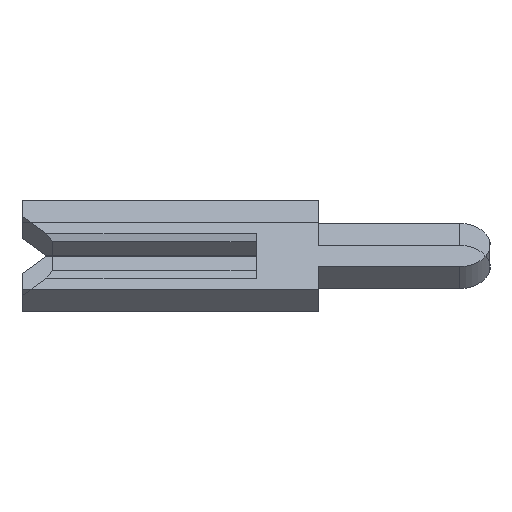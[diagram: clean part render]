
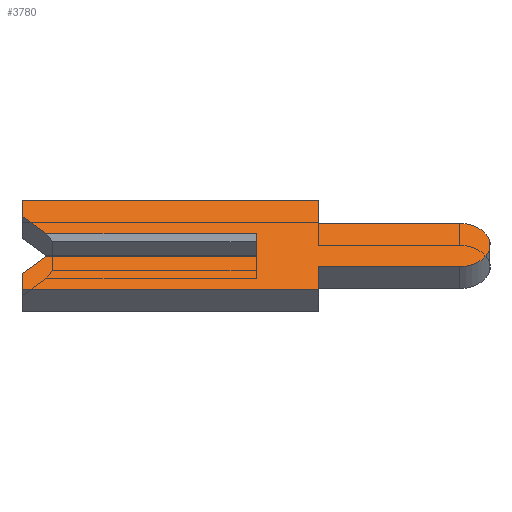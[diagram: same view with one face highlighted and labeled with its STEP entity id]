
A CAD part, left-side view. The second image highlights one B-rep face of the part: STEP entity #3780.
In plain terms, the highlighted face is planar.
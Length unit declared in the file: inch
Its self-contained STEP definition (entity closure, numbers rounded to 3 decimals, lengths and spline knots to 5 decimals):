
#26 = ORIENTED_EDGE ( 'NONE', *, *, #160, .F. ) ;
#28 = VECTOR ( 'NONE', #3910, 39.37008 ) ;
#71 = ORIENTED_EDGE ( 'NONE', *, *, #3265, .F. ) ;
#127 = ORIENTED_EDGE ( 'NONE', *, *, #2620, .F. ) ;
#139 = LINE ( 'NONE', #2826, #3987 ) ;
#149 = LINE ( 'NONE', #206, #2885 ) ;
#160 = EDGE_CURVE ( 'NONE', #2735, #2864, #1687, .T. ) ;
#175 = VECTOR ( 'NONE', #2562, 39.37008 ) ;
#206 = CARTESIAN_POINT ( 'NONE',  ( -0.01, -0.04, -0.0195 ) ) ;
#281 = CARTESIAN_POINT ( 'NONE',  ( -0.01, 0.1305, -0.0065 ) ) ;
#293 = DIRECTION ( 'NONE',  ( 0., -0.707, 0.707 ) ) ;
#316 = VERTEX_POINT ( 'NONE', #4026 ) ;
#367 = DIRECTION ( 'NONE',  ( 0., 0., -1. ) ) ;
#387 = LINE ( 'NONE', #1609, #175 ) ;
#411 = ORIENTED_EDGE ( 'NONE', *, *, #1567, .F. ) ;
#456 = VECTOR ( 'NONE', #2513, 39.37008 ) ;
#496 = VERTEX_POINT ( 'NONE', #1480 ) ;
#559 = DIRECTION ( 'NONE',  ( 0., 1., 0. ) ) ;
#669 = EDGE_CURVE ( 'NONE', #1331, #1097, #149, .T. ) ;
#706 = LINE ( 'NONE', #1332, #2945 ) ;
#759 = DIRECTION ( 'NONE',  ( 0., -1., 0. ) ) ;
#764 = EDGE_CURVE ( 'NONE', #1489, #2735, #1234, .T. ) ;
#836 = CARTESIAN_POINT ( 'NONE',  ( -0.01, -0.04, -0.04 ) ) ;
#882 = AXIS2_PLACEMENT_3D ( 'NONE', #1657, #1964, #367 ) ;
#922 = ORIENTED_EDGE ( 'NONE', *, *, #669, .F. ) ;
#923 = CARTESIAN_POINT ( 'NONE',  ( -0.01, 0.134, 0.01 ) ) ;
#948 = CARTESIAN_POINT ( 'NONE',  ( -0.01, 0., -0.01 ) ) ;
#951 = LINE ( 'NONE', #3582, #28 ) ;
#1019 = VERTEX_POINT ( 'NONE', #1838 ) ;
#1097 = VERTEX_POINT ( 'NONE', #1804 ) ;
#1100 = CARTESIAN_POINT ( 'NONE',  ( -0.01, 0.15, -0.026 ) ) ;
#1108 = LINE ( 'NONE', #1255, #3890 ) ;
#1149 = EDGE_CURVE ( 'NONE', #1521, #1019, #139, .T. ) ;
#1155 = ORIENTED_EDGE ( 'NONE', *, *, #1149, .T. ) ;
#1197 = DIRECTION ( 'NONE',  ( 0., -1., 0. ) ) ;
#1234 = LINE ( 'NONE', #3131, #1775 ) ;
#1255 = CARTESIAN_POINT ( 'NONE',  ( -0.01, 0.15, 0.04 ) ) ;
#1283 = ORIENTED_EDGE ( 'NONE', *, *, #2763, .F. ) ;
#1304 = LINE ( 'NONE', #1936, #3300 ) ;
#1317 = CARTESIAN_POINT ( 'NONE',  ( -0.01, 0.15, -0.04 ) ) ;
#1320 = VECTOR ( 'NONE', #293, 39.37008 ) ;
#1331 = VERTEX_POINT ( 'NONE', #2254 ) ;
#1332 = CARTESIAN_POINT ( 'NONE',  ( -0.01, -0.04, 0.04 ) ) ;
#1369 = DIRECTION ( 'NONE',  ( 0., 0., -1. ) ) ;
#1376 = DIRECTION ( 'NONE',  ( 0., 0., 1. ) ) ;
#1392 = EDGE_CURVE ( 'NONE', #496, #2068, #2881, .T. ) ;
#1480 = CARTESIAN_POINT ( 'NONE',  ( -0.01, 0.15, 0.026 ) ) ;
#1489 = VERTEX_POINT ( 'NONE', #836 ) ;
#1506 = EDGE_CURVE ( 'NONE', #2864, #2099, #3027, .T. ) ;
#1521 = VERTEX_POINT ( 'NONE', #923 ) ;
#1526 = CARTESIAN_POINT ( 'NONE',  ( -0.01, 0.15, 0.026 ) ) ;
#1539 = VERTEX_POINT ( 'NONE', #948 ) ;
#1567 = EDGE_CURVE ( 'NONE', #2068, #2023, #1108, .T. ) ;
#1589 = EDGE_CURVE ( 'NONE', #1097, #1489, #3474, .T. ) ;
#1609 = CARTESIAN_POINT ( 'NONE',  ( -0.01, 0.1305, 0.0065 ) ) ;
#1657 = CARTESIAN_POINT ( 'NONE',  ( -0.01, -0.1305, 0. ) ) ;
#1679 = VECTOR ( 'NONE', #2527, 39.37008 ) ;
#1687 = LINE ( 'NONE', #1100, #2042 ) ;
#1775 = VECTOR ( 'NONE', #2791, 39.37008 ) ;
#1804 = CARTESIAN_POINT ( 'NONE',  ( -0.01, -0.04, -0.0195 ) ) ;
#1817 = ORIENTED_EDGE ( 'NONE', *, *, #1506, .F. ) ;
#1837 = EDGE_CURVE ( 'NONE', #1539, #1019, #1304, .T. ) ;
#1838 = CARTESIAN_POINT ( 'NONE',  ( -0.01, 0., 0.01 ) ) ;
#1863 = EDGE_CURVE ( 'NONE', #1521, #496, #387, .T. ) ;
#1936 = CARTESIAN_POINT ( 'NONE',  ( -0.01, 0., 0.0065 ) ) ;
#1955 = DIRECTION ( 'NONE',  ( 0., 0., -1. ) ) ;
#1964 = DIRECTION ( 'NONE',  ( 1., 0., 0. ) ) ;
#1991 = CARTESIAN_POINT ( 'NONE',  ( -0.01, 0.15, -0.026 ) ) ;
#2000 = EDGE_LOOP ( 'NONE', ( #1155, #4028, #127, #1817, #26, #3494, #3516, #922, #3829, #71, #1283, #411, #2842, #3903 ) ) ;
#2023 = VERTEX_POINT ( 'NONE', #3144 ) ;
#2042 = VECTOR ( 'NONE', #4039, 39.37008 ) ;
#2068 = VERTEX_POINT ( 'NONE', #3843 ) ;
#2099 = VERTEX_POINT ( 'NONE', #2866 ) ;
#2254 = CARTESIAN_POINT ( 'NONE',  ( -0.01, -0.1305, -0.0195 ) ) ;
#2322 = AXIS2_PLACEMENT_3D ( 'NONE', #2970, #3972, #1369 ) ;
#2367 = CARTESIAN_POINT ( 'NONE',  ( -0.01, -0.04, 0.0195 ) ) ;
#2513 = DIRECTION ( 'NONE',  ( 0., 0., 1. ) ) ;
#2527 = DIRECTION ( 'NONE',  ( 0., 0., -1. ) ) ;
#2562 = DIRECTION ( 'NONE',  ( 0., 0.707, 0.707 ) ) ;
#2620 = EDGE_CURVE ( 'NONE', #2099, #1539, #951, .T. ) ;
#2735 = VERTEX_POINT ( 'NONE', #1317 ) ;
#2743 = VECTOR ( 'NONE', #759, 39.37008 ) ;
#2763 = EDGE_CURVE ( 'NONE', #2023, #2966, #706, .T. ) ;
#2791 = DIRECTION ( 'NONE',  ( 0., 1., 0. ) ) ;
#2826 = CARTESIAN_POINT ( 'NONE',  ( -0.01, 0.15, 0.01 ) ) ;
#2842 = ORIENTED_EDGE ( 'NONE', *, *, #1392, .F. ) ;
#2864 = VERTEX_POINT ( 'NONE', #1991 ) ;
#2866 = CARTESIAN_POINT ( 'NONE',  ( -0.01, 0.134, -0.01 ) ) ;
#2877 = CARTESIAN_POINT ( 'NONE',  ( -0.01, -0.04, -0.04 ) ) ;
#2881 = LINE ( 'NONE', #1526, #456 ) ;
#2885 = VECTOR ( 'NONE', #559, 39.37008 ) ;
#2904 = CARTESIAN_POINT ( 'NONE',  ( -0.01, -0.04, 0.0195 ) ) ;
#2945 = VECTOR ( 'NONE', #1955, 39.37008 ) ;
#2966 = VERTEX_POINT ( 'NONE', #2904 ) ;
#2970 = CARTESIAN_POINT ( 'NONE',  ( -0.01, -0.1305, 0. ) ) ;
#2980 = EDGE_CURVE ( 'NONE', #316, #1331, #3837, .T. ) ;
#3027 = LINE ( 'NONE', #281, #1320 ) ;
#3131 = CARTESIAN_POINT ( 'NONE',  ( -0.01, 0.15, -0.04 ) ) ;
#3144 = CARTESIAN_POINT ( 'NONE',  ( -0.01, -0.04, 0.04 ) ) ;
#3181 = DIRECTION ( 'NONE',  ( 0., -1., 0. ) ) ;
#3265 = EDGE_CURVE ( 'NONE', #2966, #316, #3588, .T. ) ;
#3300 = VECTOR ( 'NONE', #1376, 39.37008 ) ;
#3354 = FACE_OUTER_BOUND ( 'NONE', #2000, .T. ) ;
#3474 = LINE ( 'NONE', #2877, #1679 ) ;
#3494 = ORIENTED_EDGE ( 'NONE', *, *, #764, .F. ) ;
#3516 = ORIENTED_EDGE ( 'NONE', *, *, #1589, .F. ) ;
#3582 = CARTESIAN_POINT ( 'NONE',  ( -0.01, -0.1305, -0.01 ) ) ;
#3588 = LINE ( 'NONE', #2367, #2743 ) ;
#3595 = PLANE ( 'NONE',  #2322 ) ;
#3780 = ADVANCED_FACE ( 'NONE', ( #3354 ), #3595, .F. ) ;
#3829 = ORIENTED_EDGE ( 'NONE', *, *, #2980, .F. ) ;
#3837 = CIRCLE ( 'NONE', #882, 0.0195 ) ;
#3843 = CARTESIAN_POINT ( 'NONE',  ( -0.01, 0.15, 0.04 ) ) ;
#3890 = VECTOR ( 'NONE', #3181, 39.37008 ) ;
#3903 = ORIENTED_EDGE ( 'NONE', *, *, #1863, .F. ) ;
#3910 = DIRECTION ( 'NONE',  ( 0., -1., 0. ) ) ;
#3972 = DIRECTION ( 'NONE',  ( 1., 0., 0. ) ) ;
#3987 = VECTOR ( 'NONE', #1197, 39.37008 ) ;
#4026 = CARTESIAN_POINT ( 'NONE',  ( -0.01, -0.1305, 0.0195 ) ) ;
#4028 = ORIENTED_EDGE ( 'NONE', *, *, #1837, .F. ) ;
#4039 = DIRECTION ( 'NONE',  ( 0., 0., 1. ) ) ;
